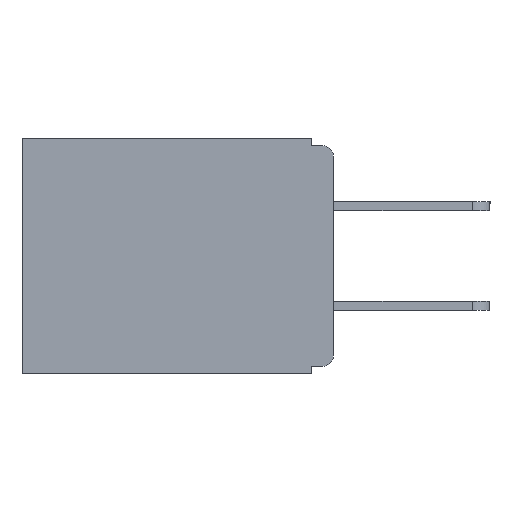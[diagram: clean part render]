
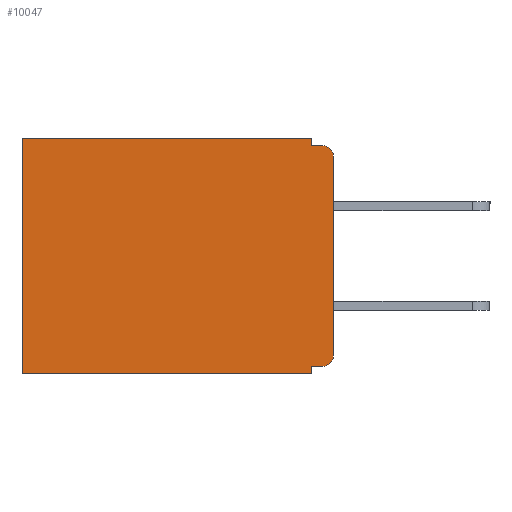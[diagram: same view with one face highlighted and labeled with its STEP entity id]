
A CAD part, left-side view. The second image highlights one B-rep face of the part: STEP entity #10047.
In plain terms, the highlighted planar face has unit normal (-1, 0, 0).
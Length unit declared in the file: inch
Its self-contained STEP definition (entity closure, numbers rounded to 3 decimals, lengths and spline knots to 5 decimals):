
#81 = EDGE_CURVE ( 'NONE', #391, #2712, #14840, .T. ) ;
#277 = ORIENTED_EDGE ( 'NONE', *, *, #10711, .T. ) ;
#307 = VECTOR ( 'NONE', #19031, 39.37008 ) ;
#384 = DIRECTION ( 'NONE',  ( -1., 0., 0. ) ) ;
#391 = VERTEX_POINT ( 'NONE', #9743 ) ;
#585 = VECTOR ( 'NONE', #18531, 39.37008 ) ;
#1280 = LINE ( 'NONE', #10999, #9236 ) ;
#1418 = CARTESIAN_POINT ( 'NONE',  ( 0.3, 0.015, -0.32 ) ) ;
#1426 = DIRECTION ( 'NONE',  ( 0., 1., 0. ) ) ;
#1464 = EDGE_CURVE ( 'NONE', #2174, #391, #15994, .T. ) ;
#1643 = DIRECTION ( 'NONE',  ( 0., 0., -1. ) ) ;
#2174 = VERTEX_POINT ( 'NONE', #8394 ) ;
#2712 = VERTEX_POINT ( 'NONE', #4622 ) ;
#3272 = VERTEX_POINT ( 'NONE', #9388 ) ;
#3496 = EDGE_CURVE ( 'NONE', #12744, #13902, #20268, .T. ) ;
#3520 = CIRCLE ( 'NONE', #20052, 0.015 ) ;
#3639 = VECTOR ( 'NONE', #15719, 39.37008 ) ;
#3968 = ORIENTED_EDGE ( 'NONE', *, *, #17746, .F. ) ;
#4622 = CARTESIAN_POINT ( 'NONE',  ( 0.3, 0.437, -0.33 ) ) ;
#4643 = DIRECTION ( 'NONE',  ( 0., 1., 0. ) ) ;
#5220 = AXIS2_PLACEMENT_3D ( 'NONE', #16733, #7254, #18297 ) ;
#5263 = EDGE_CURVE ( 'NONE', #3272, #5300, #15870, .T. ) ;
#5300 = VERTEX_POINT ( 'NONE', #8238 ) ;
#5718 = EDGE_CURVE ( 'NONE', #2174, #12744, #16348, .T. ) ;
#5947 = CARTESIAN_POINT ( 'NONE',  ( 0.3, 0.031, -0.33 ) ) ;
#6700 = ORIENTED_EDGE ( 'NONE', *, *, #81, .T. ) ;
#6751 = DIRECTION ( 'NONE',  ( 0., 0., -1. ) ) ;
#6859 = LINE ( 'NONE', #15783, #3639 ) ;
#7025 = EDGE_CURVE ( 'NONE', #18487, #2712, #6859, .T. ) ;
#7254 = DIRECTION ( 'NONE',  ( -1., 0., 0. ) ) ;
#7426 = VECTOR ( 'NONE', #12441, 39.37008 ) ;
#8200 = ORIENTED_EDGE ( 'NONE', *, *, #10321, .F. ) ;
#8238 = CARTESIAN_POINT ( 'NONE',  ( 0.3, 0., -0.305 ) ) ;
#8394 = CARTESIAN_POINT ( 'NONE',  ( 0.3, 0.031, 0. ) ) ;
#8918 = ORIENTED_EDGE ( 'NONE', *, *, #5263, .F. ) ;
#9236 = VECTOR ( 'NONE', #1426, 39.37008 ) ;
#9388 = CARTESIAN_POINT ( 'NONE',  ( 0.3, 0., -0.025 ) ) ;
#9743 = CARTESIAN_POINT ( 'NONE',  ( 0.3, 0.437, 0. ) ) ;
#9882 = CARTESIAN_POINT ( 'NONE',  ( 0.3, 0.015, -0.025 ) ) ;
#9960 = ORIENTED_EDGE ( 'NONE', *, *, #3496, .F. ) ;
#10047 = ADVANCED_FACE ( 'NONE', ( #14719 ), #15881, .F. ) ;
#10321 = EDGE_CURVE ( 'NONE', #12201, #16558, #1280, .T. ) ;
#10711 = EDGE_CURVE ( 'NONE', #12201, #5300, #14423, .T. ) ;
#10999 = CARTESIAN_POINT ( 'NONE',  ( 0.3, 0., -0.32 ) ) ;
#11148 = VECTOR ( 'NONE', #6751, 39.37008 ) ;
#11185 = VECTOR ( 'NONE', #13989, 39.37008 ) ;
#11220 = DIRECTION ( 'NONE',  ( 1., 0., 0. ) ) ;
#11513 = DIRECTION ( 'NONE',  ( 0., 0., -1. ) ) ;
#12201 = VERTEX_POINT ( 'NONE', #1418 ) ;
#12441 = DIRECTION ( 'NONE',  ( 0., 0., -1. ) ) ;
#12556 = CARTESIAN_POINT ( 'NONE',  ( 0.3, 0.031, -0.33 ) ) ;
#12744 = VERTEX_POINT ( 'NONE', #17343 ) ;
#13237 = LINE ( 'NONE', #5947, #585 ) ;
#13902 = VERTEX_POINT ( 'NONE', #20408 ) ;
#13989 = DIRECTION ( 'NONE',  ( 0., 0., -1. ) ) ;
#14073 = CARTESIAN_POINT ( 'NONE',  ( 0.3, 0.031, -0.32 ) ) ;
#14423 = CIRCLE ( 'NONE', #5220, 0.015 ) ;
#14647 = ORIENTED_EDGE ( 'NONE', *, *, #1464, .T. ) ;
#14719 = FACE_OUTER_BOUND ( 'NONE', #19155, .T. ) ;
#14840 = LINE ( 'NONE', #16972, #11148 ) ;
#15273 = CARTESIAN_POINT ( 'NONE',  ( 0.3, 0.031, 0. ) ) ;
#15479 = CARTESIAN_POINT ( 'NONE',  ( 0.3, 0., -0.33 ) ) ;
#15719 = DIRECTION ( 'NONE',  ( 0., 1., 0. ) ) ;
#15783 = CARTESIAN_POINT ( 'NONE',  ( 0.3, 0., -0.33 ) ) ;
#15870 = LINE ( 'NONE', #15479, #7426 ) ;
#15881 = PLANE ( 'NONE',  #18021 ) ;
#15994 = LINE ( 'NONE', #16707, #20113 ) ;
#16348 = LINE ( 'NONE', #15273, #11185 ) ;
#16558 = VERTEX_POINT ( 'NONE', #14073 ) ;
#16707 = CARTESIAN_POINT ( 'NONE',  ( 0.3, 0., 0. ) ) ;
#16733 = CARTESIAN_POINT ( 'NONE',  ( 0.3, 0.015, -0.305 ) ) ;
#16972 = CARTESIAN_POINT ( 'NONE',  ( 0.3, 0.437, -0.33 ) ) ;
#17330 = ORIENTED_EDGE ( 'NONE', *, *, #18060, .T. ) ;
#17343 = CARTESIAN_POINT ( 'NONE',  ( 0.3, 0.031, -0.01 ) ) ;
#17447 = CARTESIAN_POINT ( 'NONE',  ( 0.3, 0., -0.33 ) ) ;
#17746 = EDGE_CURVE ( 'NONE', #16558, #18487, #13237, .T. ) ;
#18021 = AXIS2_PLACEMENT_3D ( 'NONE', #17447, #11220, #1643 ) ;
#18060 = EDGE_CURVE ( 'NONE', #3272, #13902, #3520, .T. ) ;
#18297 = DIRECTION ( 'NONE',  ( 0., 0., -1. ) ) ;
#18302 = ORIENTED_EDGE ( 'NONE', *, *, #5718, .F. ) ;
#18487 = VERTEX_POINT ( 'NONE', #12556 ) ;
#18531 = DIRECTION ( 'NONE',  ( 0., 0., -1. ) ) ;
#18606 = CARTESIAN_POINT ( 'NONE',  ( 0.3, 0., -0.01 ) ) ;
#19031 = DIRECTION ( 'NONE',  ( 0., -1., 0. ) ) ;
#19155 = EDGE_LOOP ( 'NONE', ( #8918, #17330, #9960, #18302, #14647, #6700, #19767, #3968, #8200, #277 ) ) ;
#19767 = ORIENTED_EDGE ( 'NONE', *, *, #7025, .F. ) ;
#20052 = AXIS2_PLACEMENT_3D ( 'NONE', #9882, #384, #11513 ) ;
#20113 = VECTOR ( 'NONE', #4643, 39.37008 ) ;
#20268 = LINE ( 'NONE', #18606, #307 ) ;
#20408 = CARTESIAN_POINT ( 'NONE',  ( 0.3, 0.015, -0.01 ) ) ;
